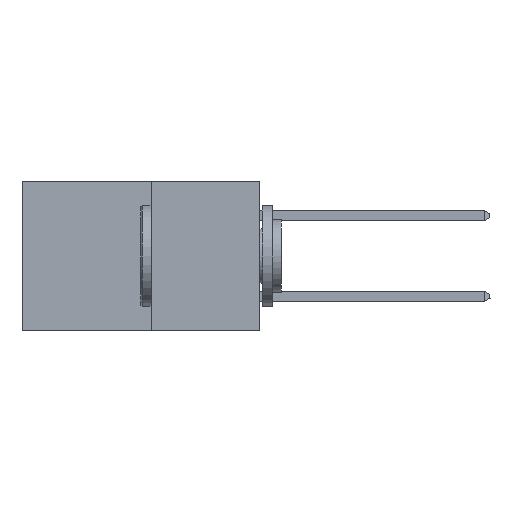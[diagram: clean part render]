
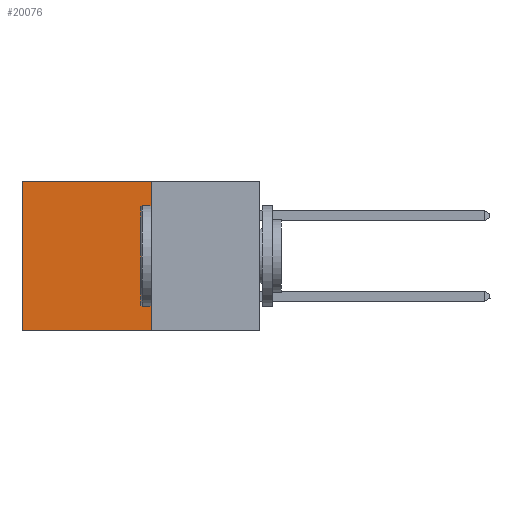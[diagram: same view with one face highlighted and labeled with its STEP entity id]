
A CAD part, left-side view. The second image highlights one B-rep face of the part: STEP entity #20076.
In plain terms, the highlighted planar face has unit normal (-1, 0, 0).
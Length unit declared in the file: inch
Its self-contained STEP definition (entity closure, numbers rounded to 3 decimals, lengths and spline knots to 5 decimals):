
#1102 = VECTOR ( 'NONE', #5325, 39.37008 ) ;
#2645 = EDGE_LOOP ( 'NONE', ( #8154, #17091, #7347, #14967 ) ) ;
#2904 = CARTESIAN_POINT ( 'NONE',  ( 0.277, 0.27, -0.37 ) ) ;
#3141 = PLANE ( 'NONE',  #15759 ) ;
#3200 = VERTEX_POINT ( 'NONE', #2904 ) ;
#3374 = VERTEX_POINT ( 'NONE', #15402 ) ;
#3441 = CARTESIAN_POINT ( 'NONE',  ( 0.277, 0.59, -0.37 ) ) ;
#5021 = CARTESIAN_POINT ( 'NONE',  ( 0.277, 0.27, -0.37 ) ) ;
#5325 = DIRECTION ( 'NONE',  ( 0., 0., -1. ) ) ;
#5490 = DIRECTION ( 'NONE',  ( 0., 1., 0. ) ) ;
#6717 = CARTESIAN_POINT ( 'NONE',  ( 0.277, 0.27, 0. ) ) ;
#6902 = DIRECTION ( 'NONE',  ( 1., 0., 0. ) ) ;
#7347 = ORIENTED_EDGE ( 'NONE', *, *, #21908, .F. ) ;
#8154 = ORIENTED_EDGE ( 'NONE', *, *, #23726, .T. ) ;
#10428 = DIRECTION ( 'NONE',  ( 0., 1., 0. ) ) ;
#10909 = LINE ( 'NONE', #6717, #20792 ) ;
#10989 = LINE ( 'NONE', #3441, #1102 ) ;
#12052 = VECTOR ( 'NONE', #5490, 39.37008 ) ;
#13959 = DIRECTION ( 'NONE',  ( 0., 0., -1. ) ) ;
#14967 = ORIENTED_EDGE ( 'NONE', *, *, #16969, .T. ) ;
#15148 = CARTESIAN_POINT ( 'NONE',  ( 0.277, 0.59, -0.37 ) ) ;
#15402 = CARTESIAN_POINT ( 'NONE',  ( 0.277, 0.27, 0. ) ) ;
#15759 = AXIS2_PLACEMENT_3D ( 'NONE', #5021, #6902, #19867 ) ;
#16969 = EDGE_CURVE ( 'NONE', #3374, #23009, #10909, .T. ) ;
#17091 = ORIENTED_EDGE ( 'NONE', *, *, #19133, .F. ) ;
#17334 = VERTEX_POINT ( 'NONE', #15148 ) ;
#18380 = CARTESIAN_POINT ( 'NONE',  ( 0.277, 0.27, -0.37 ) ) ;
#19133 = EDGE_CURVE ( 'NONE', #3200, #17334, #21909, .T. ) ;
#19867 = DIRECTION ( 'NONE',  ( 0., 0., -1. ) ) ;
#20076 = ADVANCED_FACE ( 'NONE', ( #21605 ), #3141, .F. ) ;
#20368 = VECTOR ( 'NONE', #13959, 39.37008 ) ;
#20792 = VECTOR ( 'NONE', #10428, 39.37008 ) ;
#20948 = LINE ( 'NONE', #23172, #20368 ) ;
#21605 = FACE_OUTER_BOUND ( 'NONE', #2645, .T. ) ;
#21908 = EDGE_CURVE ( 'NONE', #3374, #3200, #20948, .T. ) ;
#21909 = LINE ( 'NONE', #18380, #12052 ) ;
#23009 = VERTEX_POINT ( 'NONE', #23322 ) ;
#23172 = CARTESIAN_POINT ( 'NONE',  ( 0.277, 0.27, -0.37 ) ) ;
#23322 = CARTESIAN_POINT ( 'NONE',  ( 0.277, 0.59, 0. ) ) ;
#23726 = EDGE_CURVE ( 'NONE', #23009, #17334, #10989, .T. ) ;
